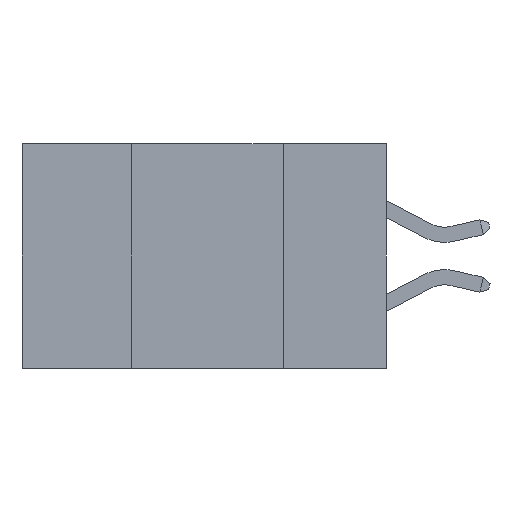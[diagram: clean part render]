
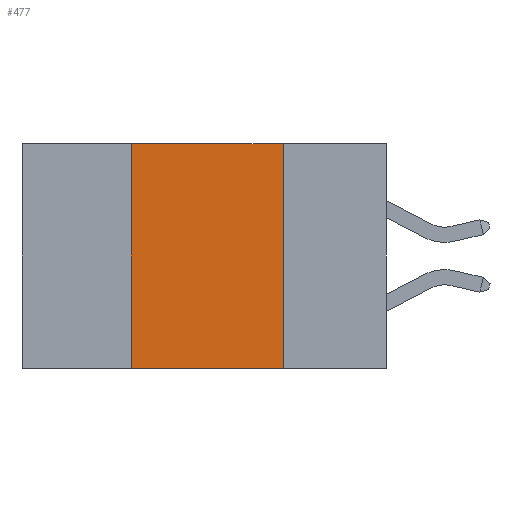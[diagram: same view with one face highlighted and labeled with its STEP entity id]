
A CAD part, left-side view. The second image highlights one B-rep face of the part: STEP entity #477.
In plain terms, the highlighted planar face has unit normal (-1, 0, 0).
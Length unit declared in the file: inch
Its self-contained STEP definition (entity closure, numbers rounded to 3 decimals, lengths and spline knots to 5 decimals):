
#16 = DIRECTION ( 'NONE',  ( 0., -1., 0. ) ) ;
#319 = DIRECTION ( 'NONE',  ( 0., 0., -1. ) ) ;
#369 = CARTESIAN_POINT ( 'NONE',  ( 0., 0.17, -0.37 ) ) ;
#477 = ADVANCED_FACE ( 'NONE', ( #2137 ), #7662, .F. ) ;
#673 = CARTESIAN_POINT ( 'NONE',  ( 0., 0.42, -0.37 ) ) ;
#782 = LINE ( 'NONE', #8037, #4278 ) ;
#899 = DIRECTION ( 'NONE',  ( 0., 0., -1. ) ) ;
#1282 = EDGE_LOOP ( 'NONE', ( #7236, #10083, #9894, #1460 ) ) ;
#1435 = DIRECTION ( 'NONE',  ( 0., -1., 0. ) ) ;
#1460 = ORIENTED_EDGE ( 'NONE', *, *, #5969, .T. ) ;
#2063 = CARTESIAN_POINT ( 'NONE',  ( 0., 0.42, -0.37 ) ) ;
#2137 = FACE_OUTER_BOUND ( 'NONE', #1282, .T. ) ;
#2160 = CARTESIAN_POINT ( 'NONE',  ( 0., 0.6, -0.37 ) ) ;
#2193 = LINE ( 'NONE', #2160, #5222 ) ;
#3404 = VERTEX_POINT ( 'NONE', #7344 ) ;
#3491 = VECTOR ( 'NONE', #16, 39.37008 ) ;
#3719 = EDGE_CURVE ( 'NONE', #4108, #3404, #7031, .T. ) ;
#4108 = VERTEX_POINT ( 'NONE', #8796 ) ;
#4278 = VECTOR ( 'NONE', #899, 39.37008 ) ;
#4482 = LINE ( 'NONE', #673, #8033 ) ;
#4539 = EDGE_CURVE ( 'NONE', #8285, #4108, #4482, .T. ) ;
#4756 = DIRECTION ( 'NONE',  ( 0., 0., 1. ) ) ;
#5118 = DIRECTION ( 'NONE',  ( 1., 0., 0. ) ) ;
#5222 = VECTOR ( 'NONE', #1435, 39.37008 ) ;
#5969 = EDGE_CURVE ( 'NONE', #8285, #8547, #2193, .T. ) ;
#6163 = AXIS2_PLACEMENT_3D ( 'NONE', #7522, #5118, #319 ) ;
#7031 = LINE ( 'NONE', #9537, #3491 ) ;
#7236 = ORIENTED_EDGE ( 'NONE', *, *, #10400, .F. ) ;
#7344 = CARTESIAN_POINT ( 'NONE',  ( 0., 0.17, 0. ) ) ;
#7522 = CARTESIAN_POINT ( 'NONE',  ( 0., 0.6, 0. ) ) ;
#7662 = PLANE ( 'NONE',  #6163 ) ;
#8033 = VECTOR ( 'NONE', #4756, 39.37008 ) ;
#8037 = CARTESIAN_POINT ( 'NONE',  ( 0., 0.17, -0.37 ) ) ;
#8285 = VERTEX_POINT ( 'NONE', #2063 ) ;
#8547 = VERTEX_POINT ( 'NONE', #369 ) ;
#8796 = CARTESIAN_POINT ( 'NONE',  ( 0., 0.42, 0. ) ) ;
#9537 = CARTESIAN_POINT ( 'NONE',  ( 0., 0.6, 0. ) ) ;
#9894 = ORIENTED_EDGE ( 'NONE', *, *, #4539, .F. ) ;
#10083 = ORIENTED_EDGE ( 'NONE', *, *, #3719, .F. ) ;
#10400 = EDGE_CURVE ( 'NONE', #3404, #8547, #782, .T. ) ;
